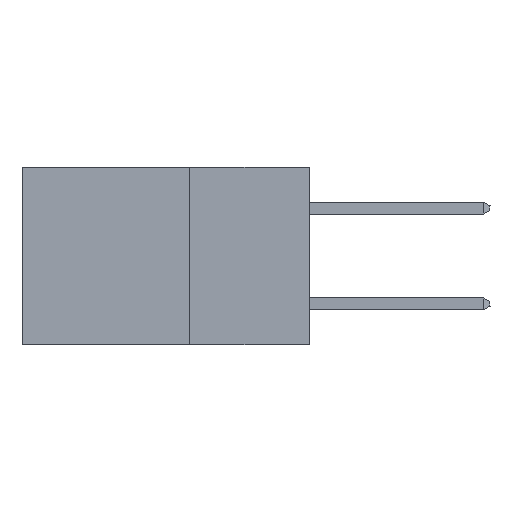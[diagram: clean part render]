
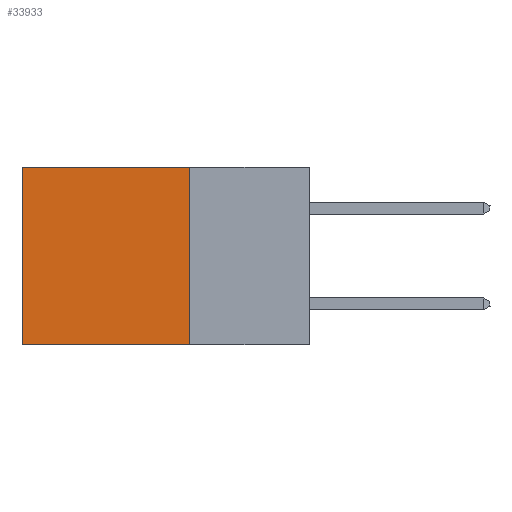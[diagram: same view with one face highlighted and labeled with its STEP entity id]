
A CAD part, left-side view. The second image highlights one B-rep face of the part: STEP entity #33933.
In plain terms, the highlighted planar face has unit normal (-1, 0, 0).
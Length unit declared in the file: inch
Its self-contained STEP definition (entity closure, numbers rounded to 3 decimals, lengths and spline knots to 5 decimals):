
#562 = EDGE_CURVE ( 'NONE', #33463, #22667, #8586, .T. ) ;
#608 = ORIENTED_EDGE ( 'NONE', *, *, #562, .F. ) ;
#3019 = LINE ( 'NONE', #35285, #25068 ) ;
#4743 = EDGE_CURVE ( 'NONE', #19600, #22667, #21500, .T. ) ;
#6171 = EDGE_LOOP ( 'NONE', ( #22924, #608, #21253, #29287 ) ) ;
#6713 = VECTOR ( 'NONE', #28621, 39.37008 ) ;
#7023 = PLANE ( 'NONE',  #11983 ) ;
#8586 = LINE ( 'NONE', #34613, #6713 ) ;
#8810 = CARTESIAN_POINT ( 'NONE',  ( 0.2875, 0.25, 0. ) ) ;
#10030 = CARTESIAN_POINT ( 'NONE',  ( 0.2875, 0.25, 0. ) ) ;
#10968 = CARTESIAN_POINT ( 'NONE',  ( 0.2875, 0.25, -0.37 ) ) ;
#11983 = AXIS2_PLACEMENT_3D ( 'NONE', #10030, #33899, #16060 ) ;
#13787 = EDGE_CURVE ( 'NONE', #22365, #33463, #3019, .T. ) ;
#14462 = DIRECTION ( 'NONE',  ( 0., 0., -1. ) ) ;
#15463 = FACE_OUTER_BOUND ( 'NONE', #6171, .T. ) ;
#16060 = DIRECTION ( 'NONE',  ( 0., 0., -1. ) ) ;
#16873 = DIRECTION ( 'NONE',  ( 0., 0., -1. ) ) ;
#17598 = DIRECTION ( 'NONE',  ( 0., 1., 0. ) ) ;
#19600 = VERTEX_POINT ( 'NONE', #20171 ) ;
#20171 = CARTESIAN_POINT ( 'NONE',  ( 0.2875, 0.6, 0. ) ) ;
#21253 = ORIENTED_EDGE ( 'NONE', *, *, #13787, .F. ) ;
#21500 = LINE ( 'NONE', #37661, #29393 ) ;
#22010 = CARTESIAN_POINT ( 'NONE',  ( 0.2875, 0.6, -0.37 ) ) ;
#22365 = VERTEX_POINT ( 'NONE', #8810 ) ;
#22667 = VERTEX_POINT ( 'NONE', #22010 ) ;
#22924 = ORIENTED_EDGE ( 'NONE', *, *, #4743, .T. ) ;
#25068 = VECTOR ( 'NONE', #14462, 39.37008 ) ;
#25687 = EDGE_CURVE ( 'NONE', #22365, #19600, #36184, .T. ) ;
#27349 = VECTOR ( 'NONE', #17598, 39.37008 ) ;
#28621 = DIRECTION ( 'NONE',  ( 0., 1., 0. ) ) ;
#29287 = ORIENTED_EDGE ( 'NONE', *, *, #25687, .T. ) ;
#29393 = VECTOR ( 'NONE', #16873, 39.37008 ) ;
#33463 = VERTEX_POINT ( 'NONE', #10968 ) ;
#33899 = DIRECTION ( 'NONE',  ( 1., 0., 0. ) ) ;
#33933 = ADVANCED_FACE ( 'NONE', ( #15463 ), #7023, .F. ) ;
#34613 = CARTESIAN_POINT ( 'NONE',  ( 0.2875, 0.25, -0.37 ) ) ;
#35285 = CARTESIAN_POINT ( 'NONE',  ( 0.2875, 0.25, 0. ) ) ;
#35385 = CARTESIAN_POINT ( 'NONE',  ( 0.2875, 0.25, 0. ) ) ;
#36184 = LINE ( 'NONE', #35385, #27349 ) ;
#37661 = CARTESIAN_POINT ( 'NONE',  ( 0.2875, 0.6, 0. ) ) ;
